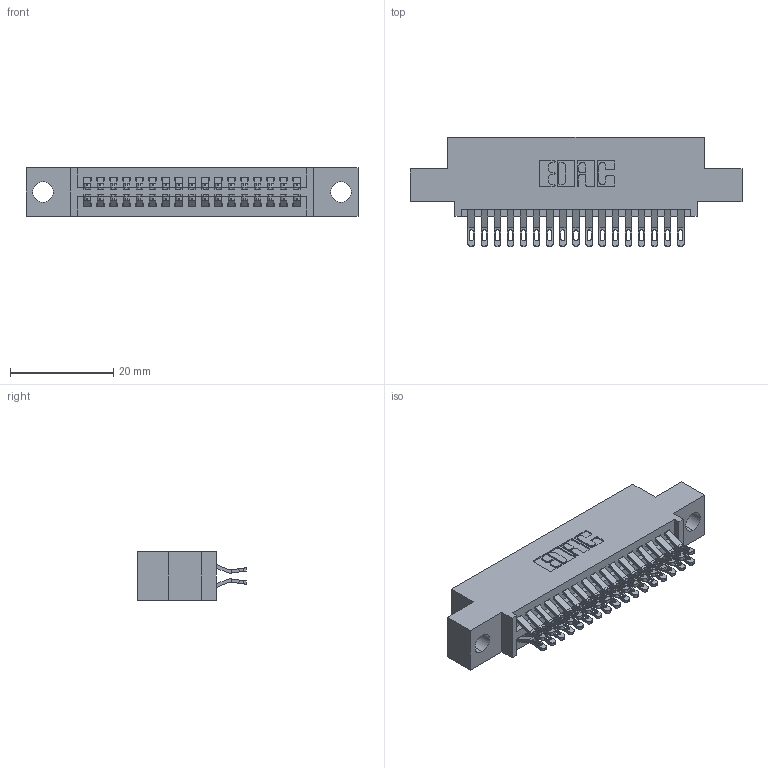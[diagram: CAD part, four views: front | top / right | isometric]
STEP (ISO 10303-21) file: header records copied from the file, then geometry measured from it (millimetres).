
FILE_DESCRIPTION (( 'STEP AP203' ), '1' );
FILE_NAME ('395-034-555-504.STEP', '2021-06-16T20:53:50', ( '' ), ( '' ), 'SwSTEP 2.0', 'SolidWorks 2020', '' );
FILE_SCHEMA (( 'CONFIG_CONTROL_DESIGN' ));
Length unit declared in the file: inch
Products named in the file (3): 345-292-001_555 Tail; 345 Part_0.110 Offset - 0.156 Dia-TI; 395-034-555-504
Assembly tree (35 placements, depth 2):
  395-034-555-504
    345 Part_0.110 Offset - 0.156 Dia-TI
    345-292-001_555 Tail  x34
Bounding box: 64.39 x 21.13 x 9.4 mm (x, y, z)
Volume: 5942.1 mm3; surface area: 8586.6 mm2
Topology: 35 solids, 35 shells, 2048 faces, 6407 edges, 4270 vertices
Faces by surface type: plane 1152, cylinder 896
Entity records: 17581 total; most frequent: CARTESIAN_POINT 3012, ORIENTED_EDGE 2914, DIRECTION 2653, EDGE_CURVE 1457, LINE 1237, VECTOR 1237, VERTEX_POINT 970, AXIS2_PLACEMENT_3D 708
